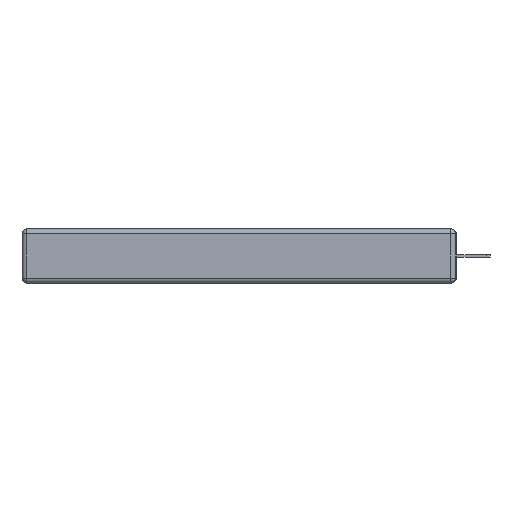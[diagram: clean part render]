
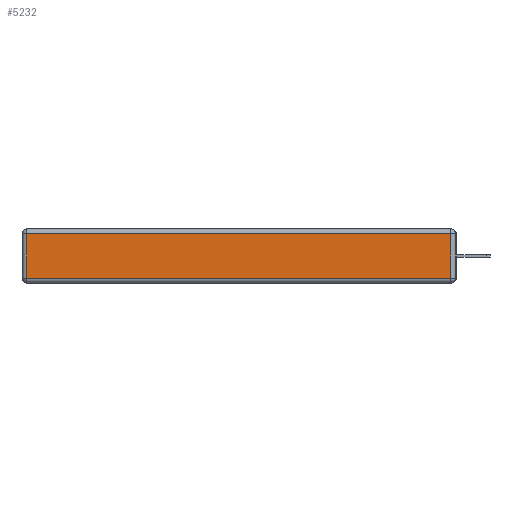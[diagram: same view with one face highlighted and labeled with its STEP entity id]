
A CAD part, left-side view. The second image highlights one B-rep face of the part: STEP entity #5232.
In plain terms, the highlighted planar face has unit normal (-1, 0, 0).
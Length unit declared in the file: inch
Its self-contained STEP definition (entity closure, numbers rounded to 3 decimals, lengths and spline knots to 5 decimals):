
#148 = VECTOR ( 'NONE', #16519, 39.37008 ) ;
#722 = VECTOR ( 'NONE', #13862, 39.37008 ) ;
#985 = VERTEX_POINT ( 'NONE', #6150 ) ;
#1106 = FACE_OUTER_BOUND ( 'NONE', #15674, .T. ) ;
#2269 = VECTOR ( 'NONE', #12747, 39.37008 ) ;
#3917 = DIRECTION ( 'NONE',  ( -1., 0., 0. ) ) ;
#4000 = VERTEX_POINT ( 'NONE', #6422 ) ;
#4086 = ORIENTED_EDGE ( 'NONE', *, *, #15785, .T. ) ;
#4318 = ORIENTED_EDGE ( 'NONE', *, *, #15878, .T. ) ;
#4365 = VERTEX_POINT ( 'NONE', #12916 ) ;
#5042 = LINE ( 'NONE', #16698, #722 ) ;
#5232 = ADVANCED_FACE ( 'NONE', ( #1106 ), #5280, .T. ) ;
#5280 = PLANE ( 'NONE',  #10010 ) ;
#6044 = VERTEX_POINT ( 'NONE', #7407 ) ;
#6150 = CARTESIAN_POINT ( 'NONE',  ( 0., 2.72, -0.313 ) ) ;
#6422 = CARTESIAN_POINT ( 'NONE',  ( 0., 0.03, -0.03 ) ) ;
#6618 = VECTOR ( 'NONE', #8397, 39.37008 ) ;
#6979 = CARTESIAN_POINT ( 'NONE',  ( 0., 2.72, -0.343 ) ) ;
#7407 = CARTESIAN_POINT ( 'NONE',  ( 0., 0.03, -0.313 ) ) ;
#8397 = DIRECTION ( 'NONE',  ( 0., 0., -1. ) ) ;
#10010 = AXIS2_PLACEMENT_3D ( 'NONE', #12417, #3917, #13879 ) ;
#10306 = LINE ( 'NONE', #18483, #2269 ) ;
#10784 = ORIENTED_EDGE ( 'NONE', *, *, #11979, .T. ) ;
#11216 = ORIENTED_EDGE ( 'NONE', *, *, #12333, .T. ) ;
#11582 = LINE ( 'NONE', #15078, #148 ) ;
#11979 = EDGE_CURVE ( 'NONE', #4000, #4365, #10306, .T. ) ;
#12333 = EDGE_CURVE ( 'NONE', #6044, #4000, #11582, .T. ) ;
#12417 = CARTESIAN_POINT ( 'NONE',  ( 0., 0., -0.343 ) ) ;
#12747 = DIRECTION ( 'NONE',  ( 0., 1., 0. ) ) ;
#12916 = CARTESIAN_POINT ( 'NONE',  ( 0., 2.72, -0.03 ) ) ;
#13862 = DIRECTION ( 'NONE',  ( 0., -1., 0. ) ) ;
#13879 = DIRECTION ( 'NONE',  ( 0., 0., 1. ) ) ;
#15078 = CARTESIAN_POINT ( 'NONE',  ( 0., 0.03, -0.343 ) ) ;
#15674 = EDGE_LOOP ( 'NONE', ( #4086, #11216, #10784, #4318 ) ) ;
#15785 = EDGE_CURVE ( 'NONE', #985, #6044, #5042, .T. ) ;
#15878 = EDGE_CURVE ( 'NONE', #4365, #985, #17989, .T. ) ;
#16519 = DIRECTION ( 'NONE',  ( 0., 0., 1. ) ) ;
#16698 = CARTESIAN_POINT ( 'NONE',  ( 0., 0., -0.313 ) ) ;
#17989 = LINE ( 'NONE', #6979, #6618 ) ;
#18483 = CARTESIAN_POINT ( 'NONE',  ( 0., 2.75, -0.03 ) ) ;
